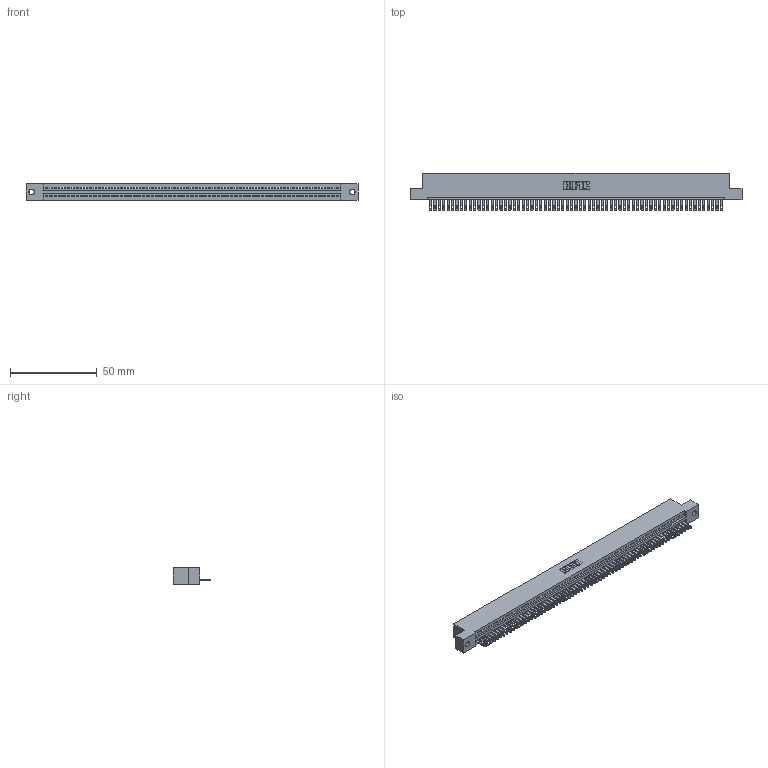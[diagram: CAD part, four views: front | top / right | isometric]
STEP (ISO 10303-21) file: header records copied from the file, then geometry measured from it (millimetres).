
FILE_DESCRIPTION (( 'STEP AP203' ), '1' );
FILE_NAME ('345-067-500-102.STEP', '2018-09-29T01:14:24', ( '' ), ( '' ), 'SwSTEP 2.0', 'SolidWorks 2016', '' );
FILE_SCHEMA (( 'CONFIG_CONTROL_DESIGN' ));
Length unit declared in the file: inch
Products named in the file (3): 345-067-500-102; 345-292-001_345-293-100; 345 Part_Flush Mounting Lugs - 0.128 Dia
Assembly tree (68 placements, depth 2):
  345-067-500-102
    345 Part_Flush Mounting Lugs - 0.128 Dia
    345-292-001_345-293-100  x67
Bounding box: 191.39 x 21.51 x 9.4 mm (x, y, z)
Volume: 18387.9 mm3; surface area: 24654.6 mm2
Topology: 68 solids, 68 shells, 3744 faces, 11597 edges, 7730 vertices
Faces by surface type: plane 2358, cylinder 1386
Entity records: 46993 total; most frequent: ORIENTED_EDGE 8146, CARTESIAN_POINT 8145, DIRECTION 7079, EDGE_CURVE 4073, VECTOR 3669, LINE 3669, VERTEX_POINT 2714, AXIS2_PLACEMENT_3D 1705
